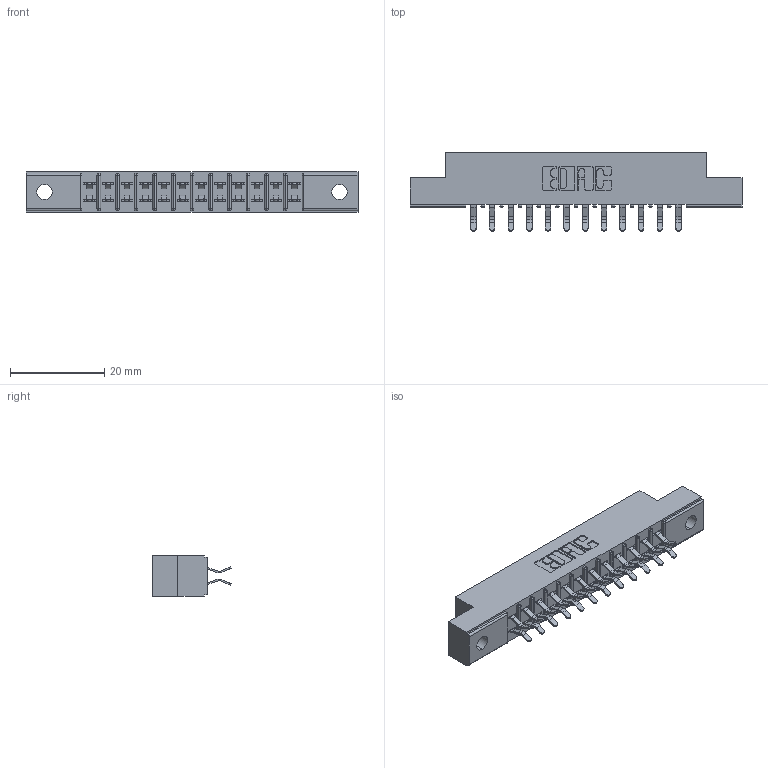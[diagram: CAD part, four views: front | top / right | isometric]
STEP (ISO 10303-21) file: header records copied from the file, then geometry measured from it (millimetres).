
FILE_DESCRIPTION (( 'STEP AP203' ), '1' );
FILE_NAME ('315-024-556-202.STEP', '2019-09-10T14:45:38', ( '' ), ( '' ), 'SwSTEP 2.0', 'SolidWorks 2016', '' );
FILE_SCHEMA (( 'CONFIG_CONTROL_DESIGN' ));
Length unit declared in the file: inch
Products named in the file (3): 315-024-556-202; 305-290-001_556; 305 Part_.128 Dia
Assembly tree (25 placements, depth 2):
  315-024-556-202
    305 Part_.128 Dia
    305-290-001_556  x24
Bounding box: 70.56 x 16.64 x 8.71 mm (x, y, z)
Volume: 4404.3 mm3; surface area: 7475.6 mm2
Topology: 25 solids, 25 shells, 1460 faces, 4192 edges, 2728 vertices
Faces by surface type: plane 812, cylinder 600, sphere 48
Entity records: 16869 total; most frequent: CARTESIAN_POINT 2794, ORIENTED_EDGE 2768, DIRECTION 2730, EDGE_CURVE 1384, VECTOR 1082, LINE 1082, VERTEX_POINT 888, AXIS2_PLACEMENT_3D 824
